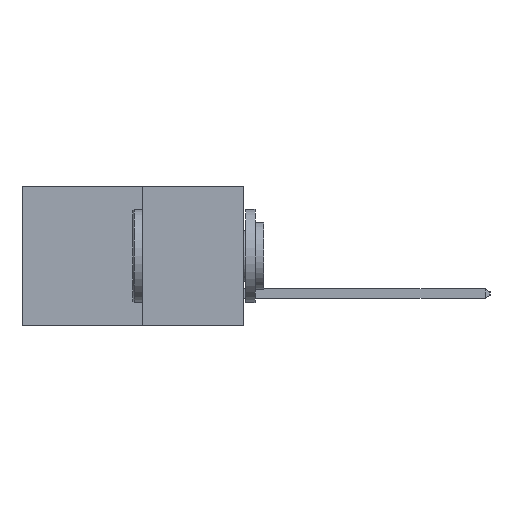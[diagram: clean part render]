
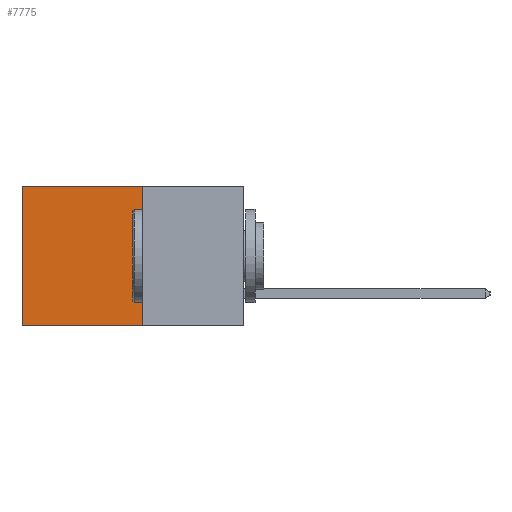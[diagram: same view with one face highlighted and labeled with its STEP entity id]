
A CAD part, left-side view. The second image highlights one B-rep face of the part: STEP entity #7775.
In plain terms, the highlighted planar face has unit normal (-1, 0, 0).
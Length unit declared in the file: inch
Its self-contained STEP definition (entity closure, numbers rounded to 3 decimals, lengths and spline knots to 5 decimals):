
#1925 = CARTESIAN_POINT ( 'NONE',  ( 0.277, 0.27, -0.37 ) ) ;
#2336 = ORIENTED_EDGE ( 'NONE', *, *, #9868, .T. ) ;
#3010 = LINE ( 'NONE', #19276, #13763 ) ;
#3748 = VERTEX_POINT ( 'NONE', #6039 ) ;
#4607 = DIRECTION ( 'NONE',  ( 0., 0., -1. ) ) ;
#4699 = CARTESIAN_POINT ( 'NONE',  ( 0.277, 0.27, -0.37 ) ) ;
#6039 = CARTESIAN_POINT ( 'NONE',  ( 0.277, 0.59, 0. ) ) ;
#6220 = EDGE_CURVE ( 'NONE', #24181, #9272, #23677, .T. ) ;
#6301 = DIRECTION ( 'NONE',  ( 0., 1., 0. ) ) ;
#6374 = DIRECTION ( 'NONE',  ( 0., 0., -1. ) ) ;
#6399 = DIRECTION ( 'NONE',  ( 1., 0., 0. ) ) ;
#6404 = PLANE ( 'NONE',  #19734 ) ;
#6894 = FACE_OUTER_BOUND ( 'NONE', #22782, .T. ) ;
#7329 = DIRECTION ( 'NONE',  ( 0., 1., 0. ) ) ;
#7405 = VECTOR ( 'NONE', #4607, 39.37008 ) ;
#7775 = ADVANCED_FACE ( 'NONE', ( #6894 ), #6404, .F. ) ;
#9272 = VERTEX_POINT ( 'NONE', #16608 ) ;
#9868 = EDGE_CURVE ( 'NONE', #3748, #9272, #18048, .T. ) ;
#9927 = CARTESIAN_POINT ( 'NONE',  ( 0.277, 0.27, -0.37 ) ) ;
#10028 = ORIENTED_EDGE ( 'NONE', *, *, #6220, .F. ) ;
#11970 = DIRECTION ( 'NONE',  ( 0., 0., -1. ) ) ;
#12722 = CARTESIAN_POINT ( 'NONE',  ( 0.277, 0.59, -0.37 ) ) ;
#13763 = VECTOR ( 'NONE', #7329, 39.37008 ) ;
#13920 = VECTOR ( 'NONE', #6301, 39.37008 ) ;
#15060 = EDGE_CURVE ( 'NONE', #19716, #3748, #3010, .T. ) ;
#16608 = CARTESIAN_POINT ( 'NONE',  ( 0.277, 0.59, -0.37 ) ) ;
#16932 = CARTESIAN_POINT ( 'NONE',  ( 0.277, 0.27, 0. ) ) ;
#17839 = VECTOR ( 'NONE', #11970, 39.37008 ) ;
#18048 = LINE ( 'NONE', #12722, #7405 ) ;
#19276 = CARTESIAN_POINT ( 'NONE',  ( 0.277, 0.27, 0. ) ) ;
#19716 = VERTEX_POINT ( 'NONE', #16932 ) ;
#19734 = AXIS2_PLACEMENT_3D ( 'NONE', #4699, #6399, #6374 ) ;
#20349 = CARTESIAN_POINT ( 'NONE',  ( 0.277, 0.27, -0.37 ) ) ;
#20893 = ORIENTED_EDGE ( 'NONE', *, *, #15060, .T. ) ;
#22288 = ORIENTED_EDGE ( 'NONE', *, *, #24016, .F. ) ;
#22782 = EDGE_LOOP ( 'NONE', ( #2336, #10028, #22288, #20893 ) ) ;
#22943 = LINE ( 'NONE', #9927, #17839 ) ;
#23677 = LINE ( 'NONE', #1925, #13920 ) ;
#24016 = EDGE_CURVE ( 'NONE', #19716, #24181, #22943, .T. ) ;
#24181 = VERTEX_POINT ( 'NONE', #20349 ) ;
